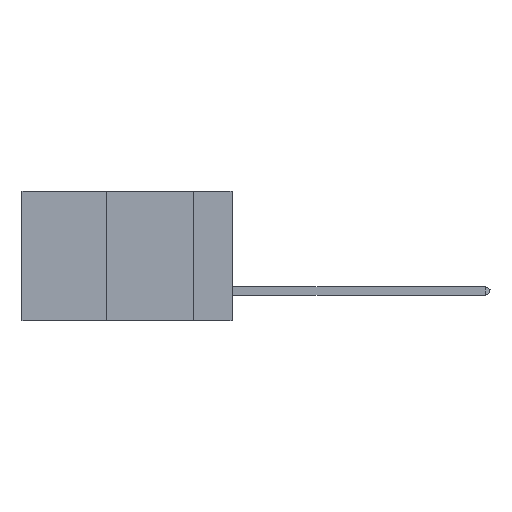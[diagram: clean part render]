
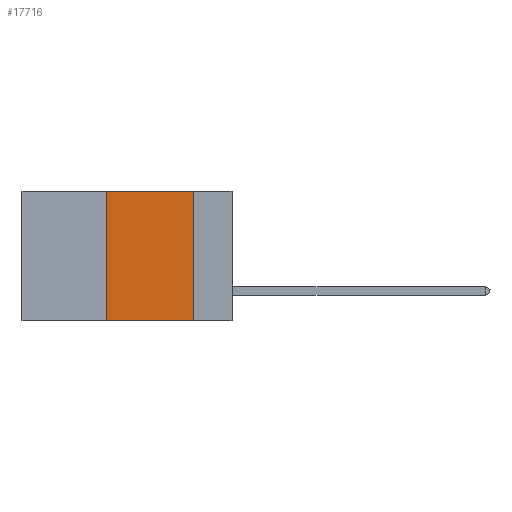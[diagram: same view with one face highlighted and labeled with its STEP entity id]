
A CAD part, left-side view. The second image highlights one B-rep face of the part: STEP entity #17716.
In plain terms, the highlighted planar face has unit normal (-1, 0, 0).
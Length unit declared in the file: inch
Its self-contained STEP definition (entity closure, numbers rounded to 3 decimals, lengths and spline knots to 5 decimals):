
#341 = CARTESIAN_POINT ( 'NONE',  ( 0., 0.6, -0.37 ) ) ;
#882 = LINE ( 'NONE', #14627, #1613 ) ;
#1613 = VECTOR ( 'NONE', #25722, 39.37008 ) ;
#2953 = CARTESIAN_POINT ( 'NONE',  ( 0., 0.11, -0.37 ) ) ;
#3186 = VECTOR ( 'NONE', #3949, 39.37008 ) ;
#3949 = DIRECTION ( 'NONE',  ( 0., -1., 0. ) ) ;
#6349 = AXIS2_PLACEMENT_3D ( 'NONE', #7694, #14681, #18290 ) ;
#7694 = CARTESIAN_POINT ( 'NONE',  ( 0., 0.6, 0. ) ) ;
#8028 = VERTEX_POINT ( 'NONE', #2953 ) ;
#9117 = VERTEX_POINT ( 'NONE', #9501 ) ;
#9501 = CARTESIAN_POINT ( 'NONE',  ( 0., 0.36, -0.37 ) ) ;
#11589 = DIRECTION ( 'NONE',  ( 0., 0., -1. ) ) ;
#12390 = VECTOR ( 'NONE', #11589, 39.37008 ) ;
#13353 = FACE_OUTER_BOUND ( 'NONE', #32547, .T. ) ;
#14627 = CARTESIAN_POINT ( 'NONE',  ( 0., 0.36, 0. ) ) ;
#14681 = DIRECTION ( 'NONE',  ( 1., 0., 0. ) ) ;
#15196 = CARTESIAN_POINT ( 'NONE',  ( 0., 0.11, 0. ) ) ;
#15447 = VERTEX_POINT ( 'NONE', #39681 ) ;
#16158 = DIRECTION ( 'NONE',  ( 0., -1., 0. ) ) ;
#16501 = EDGE_CURVE ( 'NONE', #15447, #8028, #40996, .T. ) ;
#17438 = VERTEX_POINT ( 'NONE', #45101 ) ;
#17716 = ADVANCED_FACE ( 'NONE', ( #13353 ), #26008, .F. ) ;
#18290 = DIRECTION ( 'NONE',  ( 0., 0., -1. ) ) ;
#22479 = ORIENTED_EDGE ( 'NONE', *, *, #24298, .T. ) ;
#24298 = EDGE_CURVE ( 'NONE', #9117, #8028, #25891, .T. ) ;
#25722 = DIRECTION ( 'NONE',  ( 0., 0., 1. ) ) ;
#25891 = LINE ( 'NONE', #341, #3186 ) ;
#26008 = PLANE ( 'NONE',  #6349 ) ;
#26108 = ORIENTED_EDGE ( 'NONE', *, *, #45381, .F. ) ;
#26548 = EDGE_CURVE ( 'NONE', #17438, #15447, #42666, .T. ) ;
#27967 = VECTOR ( 'NONE', #16158, 39.37008 ) ;
#31791 = ORIENTED_EDGE ( 'NONE', *, *, #26548, .F. ) ;
#32547 = EDGE_LOOP ( 'NONE', ( #36198, #31791, #26108, #22479 ) ) ;
#36198 = ORIENTED_EDGE ( 'NONE', *, *, #16501, .F. ) ;
#39055 = CARTESIAN_POINT ( 'NONE',  ( 0., 0.6, 0. ) ) ;
#39681 = CARTESIAN_POINT ( 'NONE',  ( 0., 0.11, 0. ) ) ;
#40996 = LINE ( 'NONE', #15196, #12390 ) ;
#42666 = LINE ( 'NONE', #39055, #27967 ) ;
#45101 = CARTESIAN_POINT ( 'NONE',  ( 0., 0.36, 0. ) ) ;
#45381 = EDGE_CURVE ( 'NONE', #9117, #17438, #882, .T. ) ;
